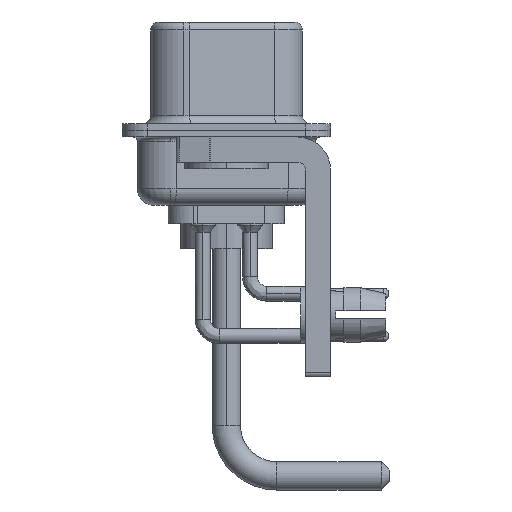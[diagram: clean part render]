
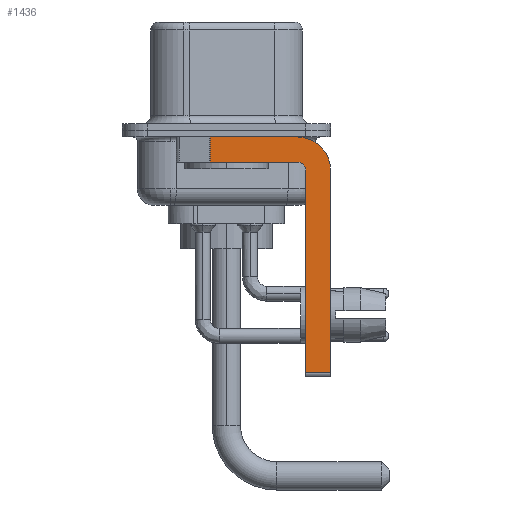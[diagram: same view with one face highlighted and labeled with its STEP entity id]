
A CAD part, left-side view. The second image highlights one B-rep face of the part: STEP entity #1436.
In plain terms, the highlighted planar face has unit normal (-1, 0, 0).
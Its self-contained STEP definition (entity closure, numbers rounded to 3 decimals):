
#334 = EDGE_CURVE ( 'NONE', #4424, #3521, #25283, .T. ) ;
#1436 = ADVANCED_FACE ( 'NONE', ( #11618 ), #7188, .F. ) ;
#1698 = EDGE_CURVE ( 'NONE', #4424, #21356, #17443, .T. ) ;
#1803 = CARTESIAN_POINT ( 'NONE',  ( -2.9, 0.978, -1.9 ) ) ;
#2001 = LINE ( 'NONE', #11026, #4269 ) ;
#2009 = CIRCLE ( 'NONE', #6162, 2. ) ;
#2121 = CARTESIAN_POINT ( 'NONE',  ( -2.9, -6.25, -2.4 ) ) ;
#2449 = VERTEX_POINT ( 'NONE', #26600 ) ;
#2505 = ORIENTED_EDGE ( 'NONE', *, *, #24198, .F. ) ;
#2528 = DIRECTION ( 'NONE',  ( 0., 1., 0. ) ) ;
#3195 = CIRCLE ( 'NONE', #12801, 0.5 ) ;
#3521 = VERTEX_POINT ( 'NONE', #20382 ) ;
#4269 = VECTOR ( 'NONE', #2528, 1000. ) ;
#4424 = VERTEX_POINT ( 'NONE', #11601 ) ;
#5730 = CARTESIAN_POINT ( 'NONE',  ( -2.9, -4.25, -2.4 ) ) ;
#5792 = CARTESIAN_POINT ( 'NONE',  ( -2.9, -4.75, -2.4 ) ) ;
#6012 = DIRECTION ( 'NONE',  ( -1., 0., 0. ) ) ;
#6162 = AXIS2_PLACEMENT_3D ( 'NONE', #26010, #10718, #14852 ) ;
#7010 = CARTESIAN_POINT ( 'NONE',  ( -2.9, -4.75, -14.8 ) ) ;
#7188 = PLANE ( 'NONE',  #12812 ) ;
#7351 = VECTOR ( 'NONE', #11285, 1000. ) ;
#7977 = DIRECTION ( 'NONE',  ( 0., 0., -1. ) ) ;
#8443 = CARTESIAN_POINT ( 'NONE',  ( -2.9, 3., -0.4 ) ) ;
#8900 = CARTESIAN_POINT ( 'NONE',  ( -2.9, -4.25, -1.9 ) ) ;
#8947 = VERTEX_POINT ( 'NONE', #5792 ) ;
#9197 = VECTOR ( 'NONE', #24015, 1000. ) ;
#10182 = CARTESIAN_POINT ( 'NONE',  ( -2.9, -4.25, -14.55 ) ) ;
#10229 = CARTESIAN_POINT ( 'NONE',  ( -2.9, -6.25, -2.4 ) ) ;
#10718 = DIRECTION ( 'NONE',  ( 1., 0., 0. ) ) ;
#10885 = ORIENTED_EDGE ( 'NONE', *, *, #23122, .F. ) ;
#11026 = CARTESIAN_POINT ( 'NONE',  ( -2.9, -4.25, -1.9 ) ) ;
#11285 = DIRECTION ( 'NONE',  ( 0., 0., 1. ) ) ;
#11485 = VECTOR ( 'NONE', #12100, 1000. ) ;
#11601 = CARTESIAN_POINT ( 'NONE',  ( -2.9, 0.978, -0.4 ) ) ;
#11618 = FACE_OUTER_BOUND ( 'NONE', #25641, .T. ) ;
#11746 = CARTESIAN_POINT ( 'NONE',  ( -2.9, -4.25, -2.4 ) ) ;
#12100 = DIRECTION ( 'NONE',  ( 0., 0., -1. ) ) ;
#12801 = AXIS2_PLACEMENT_3D ( 'NONE', #5730, #6012, #23445 ) ;
#12812 = AXIS2_PLACEMENT_3D ( 'NONE', #11746, #17768, #20471 ) ;
#13187 = EDGE_CURVE ( 'NONE', #2449, #14226, #21053, .T. ) ;
#13298 = VERTEX_POINT ( 'NONE', #8900 ) ;
#14226 = VERTEX_POINT ( 'NONE', #19698 ) ;
#14275 = ORIENTED_EDGE ( 'NONE', *, *, #1698, .F. ) ;
#14787 = ORIENTED_EDGE ( 'NONE', *, *, #13187, .T. ) ;
#14852 = DIRECTION ( 'NONE',  ( 0., 0., -1. ) ) ;
#14997 = ORIENTED_EDGE ( 'NONE', *, *, #28225, .F. ) ;
#15378 = ORIENTED_EDGE ( 'NONE', *, *, #15815, .F. ) ;
#15815 = EDGE_CURVE ( 'NONE', #17507, #14226, #20960, .T. ) ;
#17443 = LINE ( 'NONE', #8443, #9197 ) ;
#17507 = VERTEX_POINT ( 'NONE', #2121 ) ;
#17768 = DIRECTION ( 'NONE',  ( 1., 0., 0. ) ) ;
#18216 = VECTOR ( 'NONE', #18912, 1000. ) ;
#18912 = DIRECTION ( 'NONE',  ( 0., -1., 0. ) ) ;
#19698 = CARTESIAN_POINT ( 'NONE',  ( -2.9, -6.25, -14.55 ) ) ;
#20382 = CARTESIAN_POINT ( 'NONE',  ( -2.9, 0.978, -1.9 ) ) ;
#20471 = DIRECTION ( 'NONE',  ( 0., 0., -1. ) ) ;
#20960 = LINE ( 'NONE', #10229, #11485 ) ;
#21053 = LINE ( 'NONE', #10182, #18216 ) ;
#21356 = VERTEX_POINT ( 'NONE', #25640 ) ;
#21655 = ORIENTED_EDGE ( 'NONE', *, *, #334, .T. ) ;
#23122 = EDGE_CURVE ( 'NONE', #2449, #8947, #26438, .T. ) ;
#23445 = DIRECTION ( 'NONE',  ( 0., 0., 1. ) ) ;
#24015 = DIRECTION ( 'NONE',  ( 0., -1., 0. ) ) ;
#24198 = EDGE_CURVE ( 'NONE', #8947, #13298, #3195, .T. ) ;
#24961 = ORIENTED_EDGE ( 'NONE', *, *, #27436, .F. ) ;
#25067 = VECTOR ( 'NONE', #7977, 1000. ) ;
#25283 = LINE ( 'NONE', #1803, #25067 ) ;
#25640 = CARTESIAN_POINT ( 'NONE',  ( -2.9, -4.25, -0.4 ) ) ;
#25641 = EDGE_LOOP ( 'NONE', ( #14275, #21655, #24961, #2505, #10885, #14787, #15378, #14997 ) ) ;
#26010 = CARTESIAN_POINT ( 'NONE',  ( -2.9, -4.25, -2.4 ) ) ;
#26438 = LINE ( 'NONE', #7010, #7351 ) ;
#26600 = CARTESIAN_POINT ( 'NONE',  ( -2.9, -4.75, -14.55 ) ) ;
#27436 = EDGE_CURVE ( 'NONE', #13298, #3521, #2001, .T. ) ;
#28225 = EDGE_CURVE ( 'NONE', #21356, #17507, #2009, .T. ) ;
